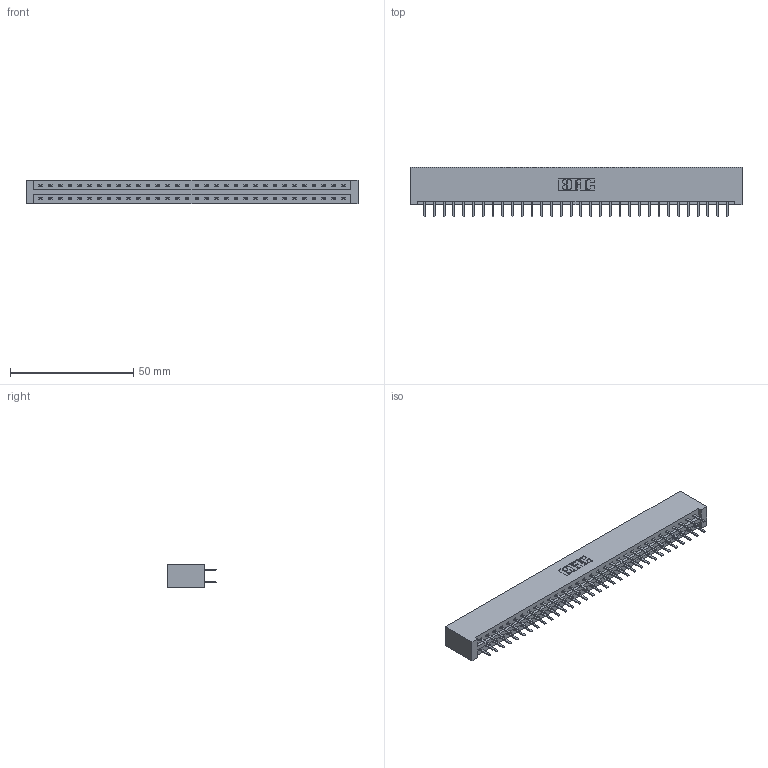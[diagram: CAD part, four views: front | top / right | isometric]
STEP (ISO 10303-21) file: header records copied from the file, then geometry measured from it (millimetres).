
FILE_DESCRIPTION (( 'STEP AP203' ), '1' );
FILE_NAME ('387-064-520-201.STEP', '2019-10-19T16:03:22', ( '' ), ( '' ), 'SwSTEP 2.0', 'SolidWorks 2016', '' );
FILE_SCHEMA (( 'CONFIG_CONTROL_DESIGN' ));
Length unit declared in the file: inch
Products named in the file (3): 387-064-520-201; 345-292-001_345-293-120; 337 Part_No Mounting Lugs
Assembly tree (65 placements, depth 2):
  387-064-520-201
    337 Part_No Mounting Lugs
    345-292-001_345-293-120  x64
Bounding box: 134.67 x 20.02 x 9.4 mm (x, y, z)
Volume: 14792.2 mm3; surface area: 16601.3 mm2
Topology: 65 solids, 65 shells, 3818 faces, 11103 edges, 7230 vertices
Faces by surface type: plane 2626, cylinder 1192
Entity records: 25941 total; most frequent: CARTESIAN_POINT 4390, ORIENTED_EDGE 4314, DIRECTION 3733, EDGE_CURVE 2157, VECTOR 2033, LINE 2033, VERTEX_POINT 1434, AXIS2_PLACEMENT_3D 850
